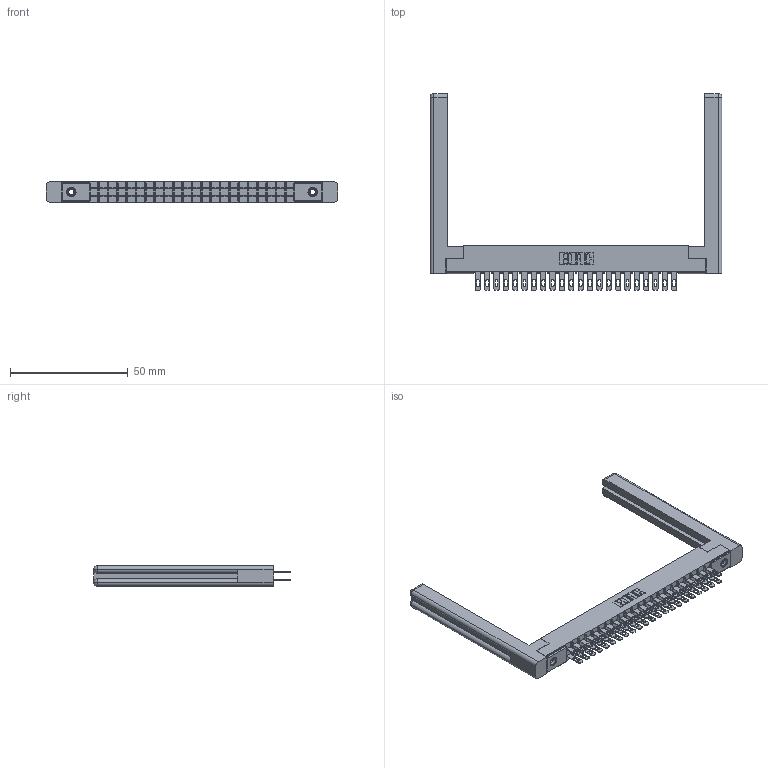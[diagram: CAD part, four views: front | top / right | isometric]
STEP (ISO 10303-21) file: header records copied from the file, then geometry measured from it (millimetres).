
FILE_DESCRIPTION (( 'STEP AP203' ), '1' );
FILE_NAME ('355-044-500-258.STEP', '2019-09-11T14:00:54', ( '' ), ( '' ), 'SwSTEP 2.0', 'SolidWorks 2016', '' );
FILE_SCHEMA (( 'CONFIG_CONTROL_DESIGN' ));
Length unit declared in the file: inch
Products named in the file (5): 345-250-001_345-250-001-102; 305 Part_.156 Dia; 355-044-500-258; 307-220-058; 305-290-001_500
Assembly tree (49 placements, depth 2):
  355-044-500-258
    305 Part_.156 Dia
    305-290-001_500  x44
    345-250-001_345-250-001-102  x2
    307-220-058  x2
Bounding box: 123.8 x 83.49 x 8.71 mm (x, y, z)
Volume: 15619.5 mm3; surface area: 20747.5 mm2
Topology: 49 solids, 49 shells, 2458 faces, 6984 edges, 4524 vertices
Faces by surface type: plane 1384, cylinder 962, sphere 88, cone 12, torus 12
Entity records: 28910 total; most frequent: CARTESIAN_POINT 4799, ORIENTED_EDGE 4702, DIRECTION 4623, EDGE_CURVE 2351, VECTOR 1867, LINE 1867, VERTEX_POINT 1500, AXIS2_PLACEMENT_3D 1378
